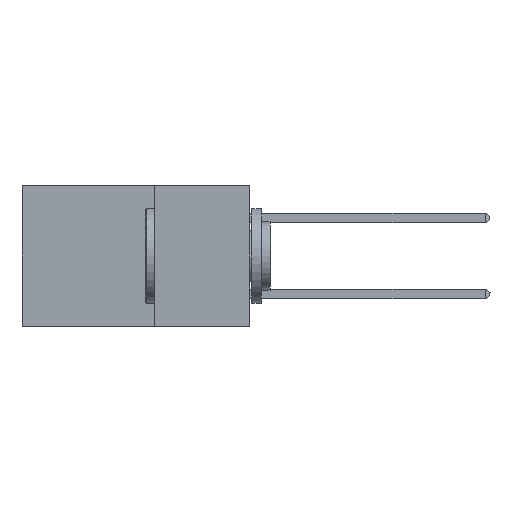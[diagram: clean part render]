
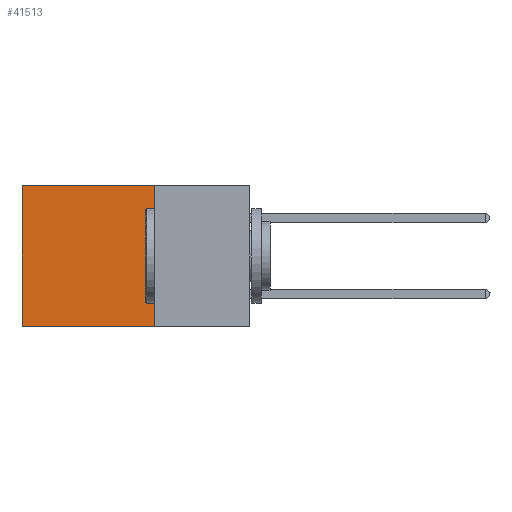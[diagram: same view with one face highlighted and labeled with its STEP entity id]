
A CAD part, left-side view. The second image highlights one B-rep face of the part: STEP entity #41513.
In plain terms, the highlighted planar face has unit normal (-1, 0, 0).
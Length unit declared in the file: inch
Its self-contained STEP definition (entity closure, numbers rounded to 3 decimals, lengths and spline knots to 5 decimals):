
#90 = VECTOR ( 'NONE', #4719, 39.37008 ) ;
#1585 = EDGE_CURVE ( 'NONE', #41902, #3287, #36334, .T. ) ;
#1611 = CARTESIAN_POINT ( 'NONE',  ( 0.2875, 0.6, -0.37 ) ) ;
#2081 = EDGE_CURVE ( 'NONE', #3287, #30878, #5383, .T. ) ;
#3287 = VERTEX_POINT ( 'NONE', #26877 ) ;
#4719 = DIRECTION ( 'NONE',  ( 0., 0., -1. ) ) ;
#4794 = LINE ( 'NONE', #31414, #35708 ) ;
#5383 = LINE ( 'NONE', #38880, #6448 ) ;
#5693 = EDGE_CURVE ( 'NONE', #9010, #30878, #4794, .T. ) ;
#6448 = VECTOR ( 'NONE', #18186, 39.37008 ) ;
#9010 = VERTEX_POINT ( 'NONE', #18113 ) ;
#10521 = ORIENTED_EDGE ( 'NONE', *, *, #5693, .T. ) ;
#11250 = CARTESIAN_POINT ( 'NONE',  ( 0.2875, 0.25, 0. ) ) ;
#12019 = ORIENTED_EDGE ( 'NONE', *, *, #1585, .F. ) ;
#12259 = DIRECTION ( 'NONE',  ( 0., 0., -1. ) ) ;
#13692 = FACE_OUTER_BOUND ( 'NONE', #34446, .T. ) ;
#18113 = CARTESIAN_POINT ( 'NONE',  ( 0.2875, 0.6, 0. ) ) ;
#18186 = DIRECTION ( 'NONE',  ( 0., 1., 0. ) ) ;
#18682 = ORIENTED_EDGE ( 'NONE', *, *, #2081, .F. ) ;
#19091 = LINE ( 'NONE', #30033, #20695 ) ;
#19803 = AXIS2_PLACEMENT_3D ( 'NONE', #35040, #21636, #12259 ) ;
#20695 = VECTOR ( 'NONE', #30899, 39.37008 ) ;
#21636 = DIRECTION ( 'NONE',  ( 1., 0., 0. ) ) ;
#24615 = DIRECTION ( 'NONE',  ( 0., 0., -1. ) ) ;
#26877 = CARTESIAN_POINT ( 'NONE',  ( 0.2875, 0.25, -0.37 ) ) ;
#30033 = CARTESIAN_POINT ( 'NONE',  ( 0.2875, 0.25, 0. ) ) ;
#30878 = VERTEX_POINT ( 'NONE', #1611 ) ;
#30899 = DIRECTION ( 'NONE',  ( 0., 1., 0. ) ) ;
#31277 = ORIENTED_EDGE ( 'NONE', *, *, #40582, .T. ) ;
#31414 = CARTESIAN_POINT ( 'NONE',  ( 0.2875, 0.6, 0. ) ) ;
#31583 = PLANE ( 'NONE',  #19803 ) ;
#34446 = EDGE_LOOP ( 'NONE', ( #10521, #18682, #12019, #31277 ) ) ;
#35040 = CARTESIAN_POINT ( 'NONE',  ( 0.2875, 0.25, 0. ) ) ;
#35708 = VECTOR ( 'NONE', #24615, 39.37008 ) ;
#36334 = LINE ( 'NONE', #11250, #90 ) ;
#38880 = CARTESIAN_POINT ( 'NONE',  ( 0.2875, 0.25, -0.37 ) ) ;
#40582 = EDGE_CURVE ( 'NONE', #41902, #9010, #19091, .T. ) ;
#41513 = ADVANCED_FACE ( 'NONE', ( #13692 ), #31583, .F. ) ;
#41902 = VERTEX_POINT ( 'NONE', #42743 ) ;
#42743 = CARTESIAN_POINT ( 'NONE',  ( 0.2875, 0.25, 0. ) ) ;
